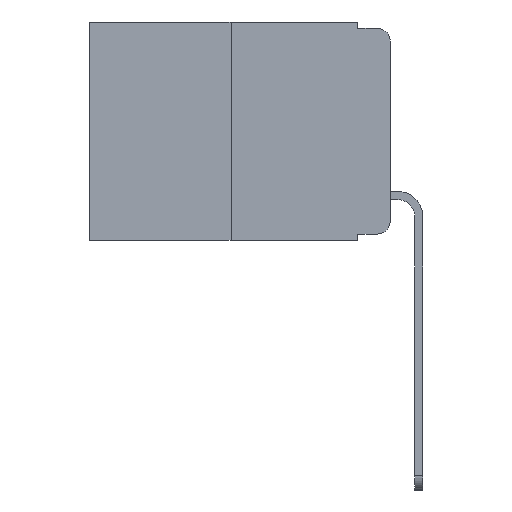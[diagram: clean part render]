
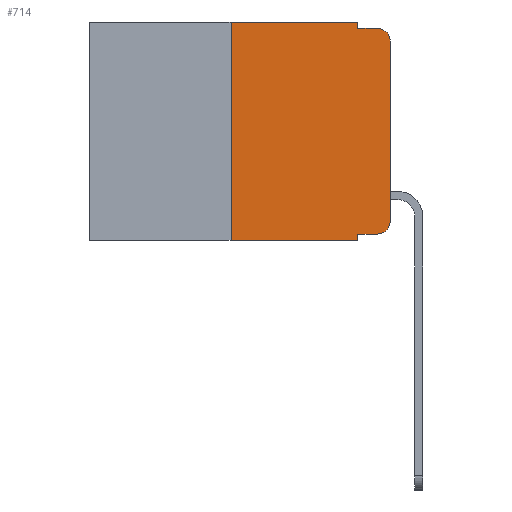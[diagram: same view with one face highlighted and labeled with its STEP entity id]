
A CAD part, left-side view. The second image highlights one B-rep face of the part: STEP entity #714.
In plain terms, the highlighted planar face has unit normal (-1, 0, 0).
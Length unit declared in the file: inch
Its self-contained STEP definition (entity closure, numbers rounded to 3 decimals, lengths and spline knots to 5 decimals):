
#643 = ORIENTED_EDGE ( 'NONE', *, *, #3048, .T. ) ;
#714 = ADVANCED_FACE ( 'NONE', ( #8691 ), #3170, .F. ) ;
#843 = DIRECTION ( 'NONE',  ( -1., 0., 0. ) ) ;
#915 = CARTESIAN_POINT ( 'NONE',  ( 0., 0.051, -0.343 ) ) ;
#1021 = VECTOR ( 'NONE', #13432, 39.37008 ) ;
#1357 = LINE ( 'NONE', #19183, #15435 ) ;
#1628 = CARTESIAN_POINT ( 'NONE',  ( 0., 0.051, 0. ) ) ;
#1992 = EDGE_CURVE ( 'NONE', #6954, #9595, #17599, .T. ) ;
#2407 = ORIENTED_EDGE ( 'NONE', *, *, #24584, .F. ) ;
#2594 = CARTESIAN_POINT ( 'NONE',  ( 0., 0.25, -0.343 ) ) ;
#2846 = VECTOR ( 'NONE', #16503, 39.37008 ) ;
#3048 = EDGE_CURVE ( 'NONE', #3609, #7247, #13948, .T. ) ;
#3170 = PLANE ( 'NONE',  #5082 ) ;
#3609 = VERTEX_POINT ( 'NONE', #22349 ) ;
#3928 = ORIENTED_EDGE ( 'NONE', *, *, #4251, .F. ) ;
#4251 = EDGE_CURVE ( 'NONE', #3609, #21429, #21975, .T. ) ;
#4287 = EDGE_CURVE ( 'NONE', #22568, #19478, #1357, .T. ) ;
#4493 = EDGE_CURVE ( 'NONE', #7247, #8851, #21109, .T. ) ;
#4531 = EDGE_CURVE ( 'NONE', #8851, #20574, #24378, .T. ) ;
#5078 = CARTESIAN_POINT ( 'NONE',  ( 0., 0.473, 0. ) ) ;
#5082 = AXIS2_PLACEMENT_3D ( 'NONE', #5078, #6916, #24057 ) ;
#5782 = LINE ( 'NONE', #22895, #6670 ) ;
#5997 = DIRECTION ( 'NONE',  ( 0., 0., -1. ) ) ;
#6117 = LINE ( 'NONE', #9588, #1021 ) ;
#6670 = VECTOR ( 'NONE', #22812, 39.37008 ) ;
#6779 = CARTESIAN_POINT ( 'NONE',  ( 0., 0.02, -0.313 ) ) ;
#6916 = DIRECTION ( 'NONE',  ( 1., 0., 0. ) ) ;
#6954 = VERTEX_POINT ( 'NONE', #21581 ) ;
#7247 = VERTEX_POINT ( 'NONE', #22571 ) ;
#7992 = EDGE_CURVE ( 'NONE', #20574, #9595, #8972, .T. ) ;
#8552 = CARTESIAN_POINT ( 'NONE',  ( 0., 0.25, 0. ) ) ;
#8691 = FACE_OUTER_BOUND ( 'NONE', #10728, .T. ) ;
#8851 = VERTEX_POINT ( 'NONE', #13612 ) ;
#8913 = CARTESIAN_POINT ( 'NONE',  ( 0., 0.051, -0.01 ) ) ;
#8972 = CIRCLE ( 'NONE', #15936, 0.02 ) ;
#9588 = CARTESIAN_POINT ( 'NONE',  ( 0., 0.473, -0.343 ) ) ;
#9595 = VERTEX_POINT ( 'NONE', #10307 ) ;
#9827 = VECTOR ( 'NONE', #18328, 39.37008 ) ;
#9845 = DIRECTION ( 'NONE',  ( 0., -1., 0. ) ) ;
#10307 = CARTESIAN_POINT ( 'NONE',  ( 0., 0.02, -0.01 ) ) ;
#10709 = CARTESIAN_POINT ( 'NONE',  ( 0., 0.051, 0. ) ) ;
#10728 = EDGE_LOOP ( 'NONE', ( #16951, #20777, #18426, #24498, #22303, #2407, #11857, #3928, #643, #20262 ) ) ;
#10914 = AXIS2_PLACEMENT_3D ( 'NONE', #6779, #843, #12320 ) ;
#11205 = EDGE_CURVE ( 'NONE', #23064, #21429, #6117, .T. ) ;
#11317 = LINE ( 'NONE', #16245, #9827 ) ;
#11698 = CARTESIAN_POINT ( 'NONE',  ( 0., 0.051, -0.333 ) ) ;
#11857 = ORIENTED_EDGE ( 'NONE', *, *, #11205, .T. ) ;
#12135 = VECTOR ( 'NONE', #17198, 39.37008 ) ;
#12320 = DIRECTION ( 'NONE',  ( 0., 0., -1. ) ) ;
#13432 = DIRECTION ( 'NONE',  ( 0., -1., 0. ) ) ;
#13612 = CARTESIAN_POINT ( 'NONE',  ( 0., 0., -0.313 ) ) ;
#13948 = LINE ( 'NONE', #11698, #15158 ) ;
#15158 = VECTOR ( 'NONE', #9845, 39.37008 ) ;
#15435 = VECTOR ( 'NONE', #21351, 39.37008 ) ;
#15936 = AXIS2_PLACEMENT_3D ( 'NONE', #22964, #19277, #5997 ) ;
#16245 = CARTESIAN_POINT ( 'NONE',  ( 0., 0.25, 0. ) ) ;
#16503 = DIRECTION ( 'NONE',  ( 0., 0., 1. ) ) ;
#16951 = ORIENTED_EDGE ( 'NONE', *, *, #4531, .T. ) ;
#17198 = DIRECTION ( 'NONE',  ( 0., 0., -1. ) ) ;
#17431 = EDGE_CURVE ( 'NONE', #19478, #6954, #5782, .T. ) ;
#17599 = LINE ( 'NONE', #8913, #23860 ) ;
#17771 = CARTESIAN_POINT ( 'NONE',  ( 0., 0., -0.03 ) ) ;
#18255 = CARTESIAN_POINT ( 'NONE',  ( 0., 0., 0. ) ) ;
#18328 = DIRECTION ( 'NONE',  ( 0., 0., 1. ) ) ;
#18426 = ORIENTED_EDGE ( 'NONE', *, *, #1992, .F. ) ;
#19183 = CARTESIAN_POINT ( 'NONE',  ( 0., 0.473, 0. ) ) ;
#19277 = DIRECTION ( 'NONE',  ( -1., 0., 0. ) ) ;
#19478 = VERTEX_POINT ( 'NONE', #10709 ) ;
#20262 = ORIENTED_EDGE ( 'NONE', *, *, #4493, .T. ) ;
#20574 = VERTEX_POINT ( 'NONE', #17771 ) ;
#20777 = ORIENTED_EDGE ( 'NONE', *, *, #7992, .T. ) ;
#20930 = DIRECTION ( 'NONE',  ( 0., -1., 0. ) ) ;
#21109 = CIRCLE ( 'NONE', #10914, 0.02 ) ;
#21351 = DIRECTION ( 'NONE',  ( 0., -1., 0. ) ) ;
#21429 = VERTEX_POINT ( 'NONE', #915 ) ;
#21581 = CARTESIAN_POINT ( 'NONE',  ( 0., 0.051, -0.01 ) ) ;
#21975 = LINE ( 'NONE', #1628, #12135 ) ;
#22303 = ORIENTED_EDGE ( 'NONE', *, *, #4287, .F. ) ;
#22349 = CARTESIAN_POINT ( 'NONE',  ( 0., 0.051, -0.333 ) ) ;
#22568 = VERTEX_POINT ( 'NONE', #8552 ) ;
#22571 = CARTESIAN_POINT ( 'NONE',  ( 0., 0.02, -0.333 ) ) ;
#22812 = DIRECTION ( 'NONE',  ( 0., 0., -1. ) ) ;
#22895 = CARTESIAN_POINT ( 'NONE',  ( 0., 0.051, 0. ) ) ;
#22964 = CARTESIAN_POINT ( 'NONE',  ( 0., 0.02, -0.03 ) ) ;
#23064 = VERTEX_POINT ( 'NONE', #2594 ) ;
#23860 = VECTOR ( 'NONE', #20930, 39.37008 ) ;
#24057 = DIRECTION ( 'NONE',  ( 0., 0., -1. ) ) ;
#24378 = LINE ( 'NONE', #18255, #2846 ) ;
#24498 = ORIENTED_EDGE ( 'NONE', *, *, #17431, .F. ) ;
#24584 = EDGE_CURVE ( 'NONE', #23064, #22568, #11317, .T. ) ;
